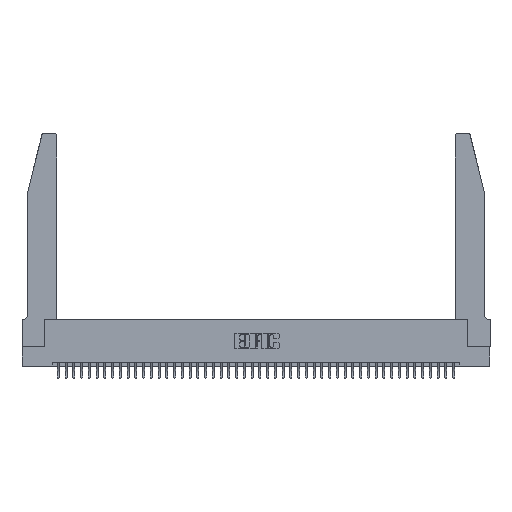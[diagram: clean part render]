
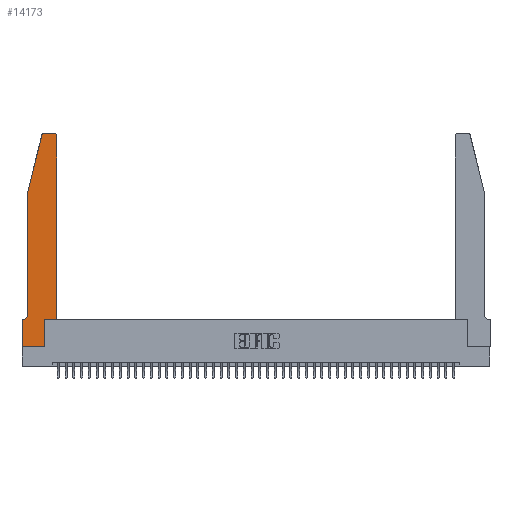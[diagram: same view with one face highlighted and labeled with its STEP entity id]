
A CAD part, top view. The second image highlights one B-rep face of the part: STEP entity #14173.
In plain terms, the highlighted planar face has unit normal (0, 0, 1).
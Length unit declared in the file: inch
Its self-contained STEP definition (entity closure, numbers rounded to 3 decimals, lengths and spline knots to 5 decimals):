
#631 = CARTESIAN_POINT ( 'NONE',  ( 0.2865, 0.35, 0.37 ) ) ;
#664 = CARTESIAN_POINT ( 'NONE',  ( 0.2605, 2.75, 0.37 ) ) ;
#817 = EDGE_CURVE ( 'NONE', #31653, #9938, #43357, .T. ) ;
#1162 = VERTEX_POINT ( 'NONE', #20615 ) ;
#1564 = LINE ( 'NONE', #30296, #27950 ) ;
#1590 = ORIENTED_EDGE ( 'NONE', *, *, #8037, .T. ) ;
#2949 = VECTOR ( 'NONE', #32726, 39.37008 ) ;
#3700 = VECTOR ( 'NONE', #28044, 39.37008 ) ;
#3860 = CARTESIAN_POINT ( 'NONE',  ( 0.284, 2.75, 0.37 ) ) ;
#4005 = CARTESIAN_POINT ( 'NONE',  ( 0.0755, 2., 0.37 ) ) ;
#4216 = DIRECTION ( 'NONE',  ( -1., 0., 0. ) ) ;
#5019 = VERTEX_POINT ( 'NONE', #10098 ) ;
#5824 = DIRECTION ( 'NONE',  ( 0., -1., 0. ) ) ;
#6413 = CARTESIAN_POINT ( 'NONE',  ( 0.2865, 0.35, 0.37 ) ) ;
#7401 = EDGE_CURVE ( 'NONE', #38453, #21109, #41968, .T. ) ;
#7537 = AXIS2_PLACEMENT_3D ( 'NONE', #11576, #35500, #15033 ) ;
#8037 = EDGE_CURVE ( 'NONE', #36379, #5019, #12159, .T. ) ;
#8598 = ORIENTED_EDGE ( 'NONE', *, *, #35159, .T. ) ;
#8827 = DIRECTION ( 'NONE',  ( 0., 0., 1. ) ) ;
#8965 = CARTESIAN_POINT ( 'NONE',  ( 0., 0., 0.37 ) ) ;
#9938 = VERTEX_POINT ( 'NONE', #40074 ) ;
#10098 = CARTESIAN_POINT ( 'NONE',  ( 0.4505, 2.72, 0.37 ) ) ;
#10570 = FACE_OUTER_BOUND ( 'NONE', #25872, .T. ) ;
#11363 = ORIENTED_EDGE ( 'NONE', *, *, #40781, .T. ) ;
#11576 = CARTESIAN_POINT ( 'NONE',  ( 0.0055, 0.42, 0.37 ) ) ;
#11678 = EDGE_CURVE ( 'NONE', #42742, #1162, #12912, .T. ) ;
#11956 = VERTEX_POINT ( 'NONE', #25935 ) ;
#12159 = LINE ( 'NONE', #25714, #2949 ) ;
#12189 = AXIS2_PLACEMENT_3D ( 'NONE', #40673, #20190, #44062 ) ;
#12530 = CARTESIAN_POINT ( 'NONE',  ( 0., 0.35, 0.37 ) ) ;
#12889 = VERTEX_POINT ( 'NONE', #35120 ) ;
#12912 = LINE ( 'NONE', #4005, #3700 ) ;
#13775 = AXIS2_PLACEMENT_3D ( 'NONE', #29328, #8827, #32771 ) ;
#13895 = CARTESIAN_POINT ( 'NONE',  ( 0., 0.35, 0.37 ) ) ;
#14173 = ADVANCED_FACE ( 'NONE', ( #10570 ), #36291, .T. ) ;
#15033 = DIRECTION ( 'NONE',  ( -1., 0., 0. ) ) ;
#15967 = DIRECTION ( 'NONE',  ( 1., 0., 0. ) ) ;
#16123 = VECTOR ( 'NONE', #36337, 39.37008 ) ;
#16739 = ORIENTED_EDGE ( 'NONE', *, *, #42329, .T. ) ;
#17200 = CARTESIAN_POINT ( 'NONE',  ( 0.25487, 2.72718, 0.37 ) ) ;
#18048 = LINE ( 'NONE', #29949, #44205 ) ;
#18254 = VERTEX_POINT ( 'NONE', #631 ) ;
#19955 = ORIENTED_EDGE ( 'NONE', *, *, #23433, .T. ) ;
#20190 = DIRECTION ( 'NONE',  ( 0., 0., 1. ) ) ;
#20414 = ORIENTED_EDGE ( 'NONE', *, *, #7401, .T. ) ;
#20511 = CARTESIAN_POINT ( 'NONE',  ( 0.4505, 0.35, 0.37 ) ) ;
#20615 = CARTESIAN_POINT ( 'NONE',  ( 0.0755, 0.42, 0.37 ) ) ;
#21109 = VERTEX_POINT ( 'NONE', #17200 ) ;
#22898 = VECTOR ( 'NONE', #23512, 39.37008 ) ;
#22908 = CARTESIAN_POINT ( 'NONE',  ( 0., 0., 0.37 ) ) ;
#23433 = EDGE_CURVE ( 'NONE', #5019, #11956, #25459, .T. ) ;
#23512 = DIRECTION ( 'NONE',  ( 0., 1., 0. ) ) ;
#24717 = LINE ( 'NONE', #22908, #42823 ) ;
#25281 = ORIENTED_EDGE ( 'NONE', *, *, #31779, .T. ) ;
#25459 = CIRCLE ( 'NONE', #12189, 0.03 ) ;
#25714 = CARTESIAN_POINT ( 'NONE',  ( 0.4505, 0.35, 0.37 ) ) ;
#25820 = LINE ( 'NONE', #28655, #42887 ) ;
#25872 = EDGE_LOOP ( 'NONE', ( #8598, #20414, #40751, #42854, #25281, #37597, #11363, #29552, #16739, #43964, #1590, #19955 ) ) ;
#25935 = CARTESIAN_POINT ( 'NONE',  ( 0.4205, 2.75, 0.37 ) ) ;
#27752 = CARTESIAN_POINT ( 'NONE',  ( 0., 0., 0.37 ) ) ;
#27950 = VECTOR ( 'NONE', #40455, 39.37008 ) ;
#28044 = DIRECTION ( 'NONE',  ( 0., -1., 0. ) ) ;
#28232 = AXIS2_PLACEMENT_3D ( 'NONE', #12530, #36448, #15967 ) ;
#28655 = CARTESIAN_POINT ( 'NONE',  ( 0.4505, 0.35, 0.37 ) ) ;
#29028 = LINE ( 'NONE', #664, #38142 ) ;
#29328 = CARTESIAN_POINT ( 'NONE',  ( 0.284, 2.72, 0.37 ) ) ;
#29552 = ORIENTED_EDGE ( 'NONE', *, *, #817, .T. ) ;
#29949 = CARTESIAN_POINT ( 'NONE',  ( 0.0755, 2., 0.37 ) ) ;
#30102 = DIRECTION ( 'NONE',  ( -0.239, -0.971, 0. ) ) ;
#30296 = CARTESIAN_POINT ( 'NONE',  ( 0.0755, 0.35, 0.37 ) ) ;
#31653 = VERTEX_POINT ( 'NONE', #27752 ) ;
#31779 = EDGE_CURVE ( 'NONE', #1162, #12889, #41392, .T. ) ;
#32004 = LINE ( 'NONE', #6413, #22898 ) ;
#32103 = DIRECTION ( 'NONE',  ( 1., 0., 0. ) ) ;
#32548 = VERTEX_POINT ( 'NONE', #13895 ) ;
#32726 = DIRECTION ( 'NONE',  ( 0., 1., 0. ) ) ;
#32771 = DIRECTION ( 'NONE',  ( 1., 0., 0. ) ) ;
#33197 = CARTESIAN_POINT ( 'NONE',  ( 0.0755, 2., 0.37 ) ) ;
#35120 = CARTESIAN_POINT ( 'NONE',  ( 0.0055, 0.35, 0.37 ) ) ;
#35159 = EDGE_CURVE ( 'NONE', #11956, #38453, #29028, .T. ) ;
#35247 = EDGE_CURVE ( 'NONE', #18254, #36379, #25820, .T. ) ;
#35500 = DIRECTION ( 'NONE',  ( 0., 0., -1. ) ) ;
#36291 = PLANE ( 'NONE',  #28232 ) ;
#36337 = DIRECTION ( 'NONE',  ( 1., 0., 0. ) ) ;
#36379 = VERTEX_POINT ( 'NONE', #20511 ) ;
#36448 = DIRECTION ( 'NONE',  ( 0., 0., 1. ) ) ;
#37597 = ORIENTED_EDGE ( 'NONE', *, *, #40232, .T. ) ;
#38142 = VECTOR ( 'NONE', #4216, 39.37008 ) ;
#38453 = VERTEX_POINT ( 'NONE', #3860 ) ;
#38899 = EDGE_CURVE ( 'NONE', #21109, #42742, #18048, .T. ) ;
#40074 = CARTESIAN_POINT ( 'NONE',  ( 0.2865, 0., 0.37 ) ) ;
#40232 = EDGE_CURVE ( 'NONE', #12889, #32548, #1564, .T. ) ;
#40455 = DIRECTION ( 'NONE',  ( -1., 0., 0. ) ) ;
#40673 = CARTESIAN_POINT ( 'NONE',  ( 0.4205, 2.72, 0.37 ) ) ;
#40751 = ORIENTED_EDGE ( 'NONE', *, *, #38899, .T. ) ;
#40781 = EDGE_CURVE ( 'NONE', #32548, #31653, #24717, .T. ) ;
#41392 = CIRCLE ( 'NONE', #7537, 0.07 ) ;
#41968 = CIRCLE ( 'NONE', #13775, 0.03 ) ;
#42329 = EDGE_CURVE ( 'NONE', #9938, #18254, #32004, .T. ) ;
#42742 = VERTEX_POINT ( 'NONE', #33197 ) ;
#42823 = VECTOR ( 'NONE', #5824, 39.37008 ) ;
#42854 = ORIENTED_EDGE ( 'NONE', *, *, #11678, .T. ) ;
#42887 = VECTOR ( 'NONE', #32103, 39.37008 ) ;
#43357 = LINE ( 'NONE', #8965, #16123 ) ;
#43964 = ORIENTED_EDGE ( 'NONE', *, *, #35247, .T. ) ;
#44062 = DIRECTION ( 'NONE',  ( 1., 0., 0. ) ) ;
#44205 = VECTOR ( 'NONE', #30102, 39.37008 ) ;
